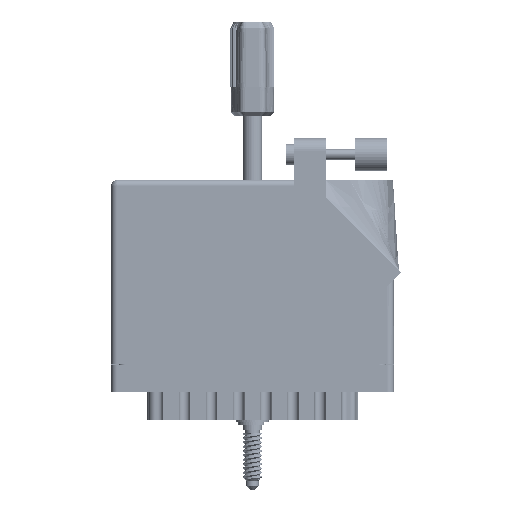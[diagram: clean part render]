
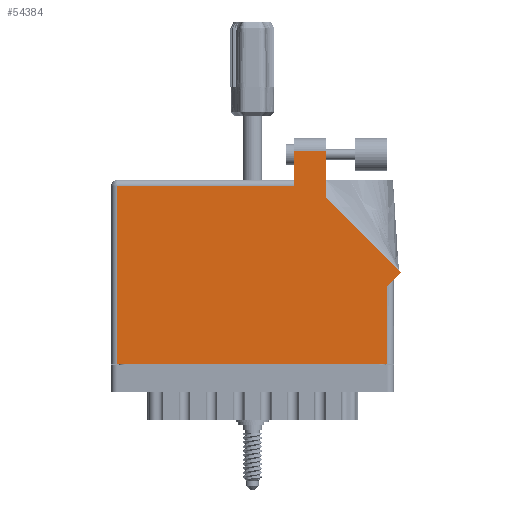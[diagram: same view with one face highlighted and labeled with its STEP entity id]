
A CAD part, front view. The second image highlights one B-rep face of the part: STEP entity #54384.
In plain terms, the highlighted face is planar.
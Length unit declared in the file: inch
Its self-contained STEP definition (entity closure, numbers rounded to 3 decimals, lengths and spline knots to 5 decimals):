
#101 = DIRECTION ( 'NONE',  ( -0.707, 0.707, 0. ) ) ;
#967 = PLANE ( 'NONE',  #57015 ) ;
#3704 = LINE ( 'NONE', #84473, #4008 ) ;
#4008 = VECTOR ( 'NONE', #11379, 39.37008 ) ;
#5004 = DIRECTION ( 'NONE',  ( 0.707, 0.707, 0. ) ) ;
#5027 = VECTOR ( 'NONE', #21144, 39.37008 ) ;
#5122 = VECTOR ( 'NONE', #85113, 39.37008 ) ;
#5574 = DIRECTION ( 'NONE',  ( 0., 1., 0. ) ) ;
#6526 = CARTESIAN_POINT ( 'NONE',  ( 1.758, 1.775, 0. ) ) ;
#9289 = EDGE_CURVE ( 'NONE', #48107, #17572, #18729, .T. ) ;
#10512 = VERTEX_POINT ( 'NONE', #71876 ) ;
#11379 = DIRECTION ( 'NONE',  ( 1., 0., 0. ) ) ;
#11382 = CARTESIAN_POINT ( 'NONE',  ( 1.758, 2.05, 0. ) ) ;
#12974 = VERTEX_POINT ( 'NONE', #71448 ) ;
#13527 = CARTESIAN_POINT ( 'NONE',  ( 1.758, 2.05, 0. ) ) ;
#13771 = DIRECTION ( 'NONE',  ( 0., -1., 0. ) ) ;
#14602 = ORIENTED_EDGE ( 'NONE', *, *, #41587, .T. ) ;
#15353 = EDGE_CURVE ( 'NONE', #30866, #48107, #89354, .T. ) ;
#16922 = VERTEX_POINT ( 'NONE', #81583 ) ;
#17572 = VERTEX_POINT ( 'NONE', #79577 ) ;
#18595 = LINE ( 'NONE', #39857, #63492 ) ;
#18729 = LINE ( 'NONE', #67622, #51039 ) ;
#19183 = CARTESIAN_POINT ( 'NONE',  ( 2.78871, 0.88571, 0. ) ) ;
#20872 = VERTEX_POINT ( 'NONE', #83833 ) ;
#21144 = DIRECTION ( 'NONE',  ( 0., -1., 0. ) ) ;
#21740 = VERTEX_POINT ( 'NONE', #11382 ) ;
#21803 = LINE ( 'NONE', #57127, #72853 ) ;
#22301 = ORIENTED_EDGE ( 'NONE', *, *, #71782, .T. ) ;
#22685 = DIRECTION ( 'NONE',  ( 0., 0., -1. ) ) ;
#26863 = ORIENTED_EDGE ( 'NONE', *, *, #47075, .T. ) ;
#27169 = ORIENTED_EDGE ( 'NONE', *, *, #38555, .T. ) ;
#29021 = FACE_OUTER_BOUND ( 'NONE', #65050, .T. ) ;
#29193 = ORIENTED_EDGE ( 'NONE', *, *, #9289, .T. ) ;
#29418 = CARTESIAN_POINT ( 'NONE',  ( 2.78871, 0.88571, 0. ) ) ;
#29580 = EDGE_CURVE ( 'NONE', #16922, #12974, #50253, .T. ) ;
#30866 = VERTEX_POINT ( 'NONE', #29418 ) ;
#31976 = EDGE_CURVE ( 'NONE', #10512, #16922, #3704, .T. ) ;
#33007 = LINE ( 'NONE', #13527, #64119 ) ;
#38555 = EDGE_CURVE ( 'NONE', #20872, #68821, #21803, .T. ) ;
#39857 = CARTESIAN_POINT ( 'NONE',  ( 2.718, 0.815, 0. ) ) ;
#41587 = EDGE_CURVE ( 'NONE', #68821, #10512, #69581, .T. ) ;
#42653 = DIRECTION ( 'NONE',  ( -1., 0., 0. ) ) ;
#44987 = CARTESIAN_POINT ( 'NONE',  ( 2.065, 1.60942, 0. ) ) ;
#47075 = EDGE_CURVE ( 'NONE', #12974, #30866, #18595, .T. ) ;
#48107 = VERTEX_POINT ( 'NONE', #44987 ) ;
#49420 = DIRECTION ( 'NONE',  ( -1., 0., 0. ) ) ;
#49935 = ORIENTED_EDGE ( 'NONE', *, *, #69470, .T. ) ;
#50253 = LINE ( 'NONE', #86001, #5122 ) ;
#51039 = VECTOR ( 'NONE', #5574, 39.37008 ) ;
#51553 = ORIENTED_EDGE ( 'NONE', *, *, #15353, .T. ) ;
#54384 = ADVANCED_FACE ( 'NONE', ( #29021 ), #967, .F. ) ;
#57015 = AXIS2_PLACEMENT_3D ( 'NONE', #83839, #22685, #49420 ) ;
#57127 = CARTESIAN_POINT ( 'NONE',  ( 0., 1.713, 0. ) ) ;
#57392 = ORIENTED_EDGE ( 'NONE', *, *, #29580, .T. ) ;
#58604 = VECTOR ( 'NONE', #101, 39.37008 ) ;
#61878 = CARTESIAN_POINT ( 'NONE',  ( 0.062, 0., 0. ) ) ;
#62302 = VECTOR ( 'NONE', #13771, 39.37008 ) ;
#63492 = VECTOR ( 'NONE', #5004, 39.37008 ) ;
#64119 = VECTOR ( 'NONE', #74240, 39.37008 ) ;
#65050 = EDGE_LOOP ( 'NONE', ( #29193, #49935, #22301, #27169, #14602, #86881, #57392, #26863, #51553 ) ) ;
#67622 = CARTESIAN_POINT ( 'NONE',  ( 2.065, 1.60942, 0. ) ) ;
#67671 = LINE ( 'NONE', #6526, #62302 ) ;
#68821 = VERTEX_POINT ( 'NONE', #80245 ) ;
#69470 = EDGE_CURVE ( 'NONE', #17572, #21740, #33007, .T. ) ;
#69581 = LINE ( 'NONE', #61878, #5027 ) ;
#71448 = CARTESIAN_POINT ( 'NONE',  ( 2.656, 0.753, 0. ) ) ;
#71782 = EDGE_CURVE ( 'NONE', #21740, #20872, #67671, .T. ) ;
#71876 = CARTESIAN_POINT ( 'NONE',  ( 0.062, 0., 0. ) ) ;
#72853 = VECTOR ( 'NONE', #42653, 39.37008 ) ;
#74240 = DIRECTION ( 'NONE',  ( -1., 0., 0. ) ) ;
#79577 = CARTESIAN_POINT ( 'NONE',  ( 2.065, 2.05, 0. ) ) ;
#80245 = CARTESIAN_POINT ( 'NONE',  ( 0.062, 1.713, 0. ) ) ;
#81583 = CARTESIAN_POINT ( 'NONE',  ( 2.656, 0., 0. ) ) ;
#83833 = CARTESIAN_POINT ( 'NONE',  ( 1.758, 1.713, 0. ) ) ;
#83839 = CARTESIAN_POINT ( 'NONE',  ( 0., 1.775, 0. ) ) ;
#84473 = CARTESIAN_POINT ( 'NONE',  ( 0., 0., 0. ) ) ;
#85113 = DIRECTION ( 'NONE',  ( 0., 1., 0. ) ) ;
#86001 = CARTESIAN_POINT ( 'NONE',  ( 2.656, 0.815, 0. ) ) ;
#86881 = ORIENTED_EDGE ( 'NONE', *, *, #31976, .T. ) ;
#89354 = LINE ( 'NONE', #19183, #58604 ) ;
